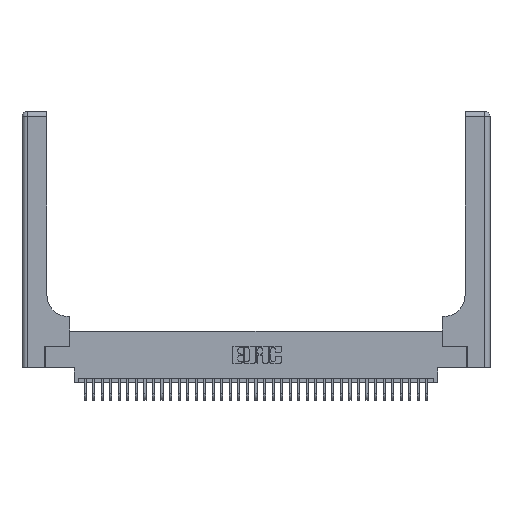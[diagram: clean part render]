
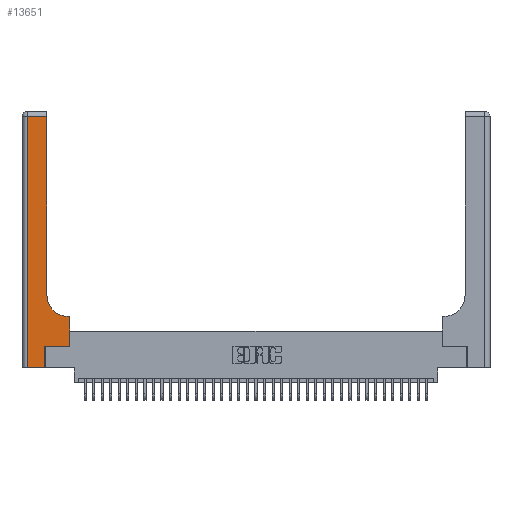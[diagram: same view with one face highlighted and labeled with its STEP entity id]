
A CAD part, top view. The second image highlights one B-rep face of the part: STEP entity #13651.
In plain terms, the highlighted planar face has unit normal (0, 0, 1).
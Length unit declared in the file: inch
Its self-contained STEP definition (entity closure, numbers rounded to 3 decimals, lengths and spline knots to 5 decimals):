
#1493 = CARTESIAN_POINT ( 'NONE',  ( 0.5585, 0.6, 0.37 ) ) ;
#1645 = LINE ( 'NONE', #30122, #23926 ) ;
#1847 = LINE ( 'NONE', #15633, #8984 ) ;
#2048 = VERTEX_POINT ( 'NONE', #5416 ) ;
#2078 = ORIENTED_EDGE ( 'NONE', *, *, #36657, .T. ) ;
#2118 = ORIENTED_EDGE ( 'NONE', *, *, #16699, .T. ) ;
#2773 = DIRECTION ( 'NONE',  ( 0., 0., -1. ) ) ;
#3015 = EDGE_CURVE ( 'NONE', #10953, #26058, #4124, .T. ) ;
#3934 = CARTESIAN_POINT ( 'NONE',  ( 0.5585, 0.25, 0.37 ) ) ;
#4124 = LINE ( 'NONE', #22857, #37782 ) ;
#4249 = DIRECTION ( 'NONE',  ( 1., 0., 0. ) ) ;
#5416 = CARTESIAN_POINT ( 'NONE',  ( 0.2915, 0.85, 0.37 ) ) ;
#5551 = CARTESIAN_POINT ( 'NONE',  ( 0.2915, 3., 0.37 ) ) ;
#6873 = ORIENTED_EDGE ( 'NONE', *, *, #15804, .T. ) ;
#7811 = CARTESIAN_POINT ( 'NONE',  ( 0.06, 2.94, 0.37 ) ) ;
#8982 = CARTESIAN_POINT ( 'NONE',  ( 0.2915, 2.94, 0.37 ) ) ;
#8984 = VECTOR ( 'NONE', #18807, 39.37008 ) ;
#10184 = LINE ( 'NONE', #34572, #25295 ) ;
#10953 = VERTEX_POINT ( 'NONE', #30268 ) ;
#12035 = DIRECTION ( 'NONE',  ( 0., 1., 0. ) ) ;
#12239 = VECTOR ( 'NONE', #29943, 39.37008 ) ;
#12352 = CARTESIAN_POINT ( 'NONE',  ( 0.269, 0.25, 0.37 ) ) ;
#13651 = ADVANCED_FACE ( 'NONE', ( #28381 ), #33210, .F. ) ;
#13990 = AXIS2_PLACEMENT_3D ( 'NONE', #39200, #2773, #21172 ) ;
#14351 = EDGE_CURVE ( 'NONE', #36276, #29357, #36860, .T. ) ;
#14972 = ORIENTED_EDGE ( 'NONE', *, *, #14351, .T. ) ;
#15139 = LINE ( 'NONE', #15636, #21784 ) ;
#15633 = CARTESIAN_POINT ( 'NONE',  ( 0.269, 0.25, 0.37 ) ) ;
#15636 = CARTESIAN_POINT ( 'NONE',  ( 0., 2.94, 0.37 ) ) ;
#15804 = EDGE_CURVE ( 'NONE', #26318, #17341, #1645, .T. ) ;
#16189 = DIRECTION ( 'NONE',  ( 0., 1., 0. ) ) ;
#16699 = EDGE_CURVE ( 'NONE', #18762, #36276, #21559, .T. ) ;
#17341 = VERTEX_POINT ( 'NONE', #36199 ) ;
#18762 = VERTEX_POINT ( 'NONE', #3934 ) ;
#18807 = DIRECTION ( 'NONE',  ( 1., 0., 0. ) ) ;
#19612 = AXIS2_PLACEMENT_3D ( 'NONE', #33937, #30893, #30768 ) ;
#19842 = CIRCLE ( 'NONE', #19612, 0.25 ) ;
#21172 = DIRECTION ( 'NONE',  ( -1., 0., 0. ) ) ;
#21559 = LINE ( 'NONE', #32628, #25797 ) ;
#21784 = VECTOR ( 'NONE', #30981, 39.37008 ) ;
#22857 = CARTESIAN_POINT ( 'NONE',  ( 0.269, 0., 0.37 ) ) ;
#23926 = VECTOR ( 'NONE', #27425, 39.37008 ) ;
#24040 = ORIENTED_EDGE ( 'NONE', *, *, #28552, .T. ) ;
#25295 = VECTOR ( 'NONE', #4249, 39.37008 ) ;
#25797 = VECTOR ( 'NONE', #28103, 39.37008 ) ;
#26058 = VERTEX_POINT ( 'NONE', #12352 ) ;
#26318 = VERTEX_POINT ( 'NONE', #7811 ) ;
#26705 = ORIENTED_EDGE ( 'NONE', *, *, #38788, .T. ) ;
#27260 = CARTESIAN_POINT ( 'NONE',  ( 0.2915, 0.6, 0.37 ) ) ;
#27425 = DIRECTION ( 'NONE',  ( 0., -1., 0. ) ) ;
#27746 = EDGE_CURVE ( 'NONE', #2048, #37742, #36537, .T. ) ;
#28012 = ORIENTED_EDGE ( 'NONE', *, *, #3015, .T. ) ;
#28103 = DIRECTION ( 'NONE',  ( 0., 1., 0. ) ) ;
#28381 = FACE_OUTER_BOUND ( 'NONE', #35314, .T. ) ;
#28552 = EDGE_CURVE ( 'NONE', #29357, #2048, #19842, .T. ) ;
#28713 = ORIENTED_EDGE ( 'NONE', *, *, #27746, .T. ) ;
#29173 = ORIENTED_EDGE ( 'NONE', *, *, #30669, .T. ) ;
#29357 = VERTEX_POINT ( 'NONE', #34816 ) ;
#29408 = VECTOR ( 'NONE', #12035, 39.37008 ) ;
#29943 = DIRECTION ( 'NONE',  ( -1., 0., 0. ) ) ;
#30122 = CARTESIAN_POINT ( 'NONE',  ( 0.06, 3., 0.37 ) ) ;
#30268 = CARTESIAN_POINT ( 'NONE',  ( 0.269, 0., 0.37 ) ) ;
#30669 = EDGE_CURVE ( 'NONE', #26058, #18762, #1847, .T. ) ;
#30768 = DIRECTION ( 'NONE',  ( 1., 0., 0. ) ) ;
#30893 = DIRECTION ( 'NONE',  ( 0., 0., -1. ) ) ;
#30981 = DIRECTION ( 'NONE',  ( -1., 0., 0. ) ) ;
#32628 = CARTESIAN_POINT ( 'NONE',  ( 0.5585, 0.25, 0.37 ) ) ;
#33210 = PLANE ( 'NONE',  #13990 ) ;
#33937 = CARTESIAN_POINT ( 'NONE',  ( 0.5415, 0.85, 0.37 ) ) ;
#34572 = CARTESIAN_POINT ( 'NONE',  ( 0., 0., 0.37 ) ) ;
#34816 = CARTESIAN_POINT ( 'NONE',  ( 0.5415, 0.6, 0.37 ) ) ;
#35314 = EDGE_LOOP ( 'NONE', ( #28713, #2078, #6873, #26705, #28012, #29173, #2118, #14972, #24040 ) ) ;
#36199 = CARTESIAN_POINT ( 'NONE',  ( 0.06, 0., 0.37 ) ) ;
#36276 = VERTEX_POINT ( 'NONE', #1493 ) ;
#36537 = LINE ( 'NONE', #5551, #29408 ) ;
#36657 = EDGE_CURVE ( 'NONE', #37742, #26318, #15139, .T. ) ;
#36860 = LINE ( 'NONE', #27260, #12239 ) ;
#37742 = VERTEX_POINT ( 'NONE', #8982 ) ;
#37782 = VECTOR ( 'NONE', #16189, 39.37008 ) ;
#38788 = EDGE_CURVE ( 'NONE', #17341, #10953, #10184, .T. ) ;
#39200 = CARTESIAN_POINT ( 'NONE',  ( 0., 3., 0.37 ) ) ;
